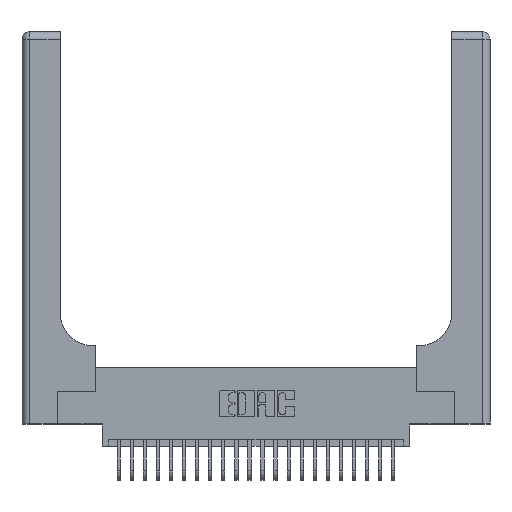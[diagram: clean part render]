
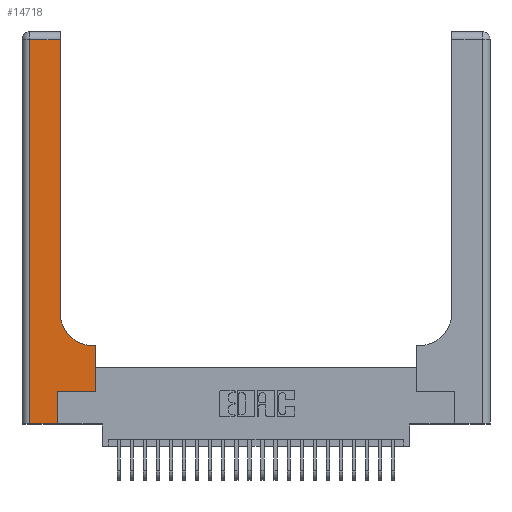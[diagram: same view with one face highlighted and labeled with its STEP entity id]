
A CAD part, top view. The second image highlights one B-rep face of the part: STEP entity #14718.
In plain terms, the highlighted planar face has unit normal (0, 0, 1).
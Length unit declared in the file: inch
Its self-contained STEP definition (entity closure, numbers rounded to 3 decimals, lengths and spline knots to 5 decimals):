
#81 = EDGE_CURVE ( 'NONE', #1444, #2046, #4703, .T. ) ;
#91 = VERTEX_POINT ( 'NONE', #6075 ) ;
#404 = VERTEX_POINT ( 'NONE', #10961 ) ;
#460 = AXIS2_PLACEMENT_3D ( 'NONE', #19530, #2668, #13280 ) ;
#1037 = ORIENTED_EDGE ( 'NONE', *, *, #14187, .T. ) ;
#1044 = FACE_OUTER_BOUND ( 'NONE', #12838, .T. ) ;
#1063 = ORIENTED_EDGE ( 'NONE', *, *, #23342, .T. ) ;
#1372 = CARTESIAN_POINT ( 'NONE',  ( 0., 0., 0.37 ) ) ;
#1444 = VERTEX_POINT ( 'NONE', #19657 ) ;
#1513 = DIRECTION ( 'NONE',  ( 1., 0., 0. ) ) ;
#2046 = VERTEX_POINT ( 'NONE', #17172 ) ;
#2134 = VECTOR ( 'NONE', #10286, 39.37008 ) ;
#2164 = ORIENTED_EDGE ( 'NONE', *, *, #81, .T. ) ;
#2668 = DIRECTION ( 'NONE',  ( 0., 0., -1. ) ) ;
#2847 = CARTESIAN_POINT ( 'NONE',  ( 0.269, 0.25, 0.37 ) ) ;
#3532 = VECTOR ( 'NONE', #17425, 39.37008 ) ;
#4218 = LINE ( 'NONE', #2847, #19525 ) ;
#4459 = ORIENTED_EDGE ( 'NONE', *, *, #10634, .T. ) ;
#4656 = LINE ( 'NONE', #13996, #14428 ) ;
#4703 = LINE ( 'NONE', #25936, #19701 ) ;
#5780 = EDGE_CURVE ( 'NONE', #404, #91, #26112, .T. ) ;
#6016 = CARTESIAN_POINT ( 'NONE',  ( 0.2915, 0.85, 0.37 ) ) ;
#6075 = CARTESIAN_POINT ( 'NONE',  ( 0.06, 2.94, 0.37 ) ) ;
#6311 = PLANE ( 'NONE',  #460 ) ;
#7303 = CARTESIAN_POINT ( 'NONE',  ( 0.2915, 3., 0.37 ) ) ;
#7791 = DIRECTION ( 'NONE',  ( 0., 1., 0. ) ) ;
#9221 = ORIENTED_EDGE ( 'NONE', *, *, #11347, .T. ) ;
#9480 = CARTESIAN_POINT ( 'NONE',  ( 0., 2.94, 0.37 ) ) ;
#9485 = AXIS2_PLACEMENT_3D ( 'NONE', #26447, #13960, #1513 ) ;
#10286 = DIRECTION ( 'NONE',  ( 0., 1., 0. ) ) ;
#10455 = CARTESIAN_POINT ( 'NONE',  ( 0.269, 0., 0.37 ) ) ;
#10634 = EDGE_CURVE ( 'NONE', #19384, #22992, #16503, .T. ) ;
#10961 = CARTESIAN_POINT ( 'NONE',  ( 0.2915, 2.94, 0.37 ) ) ;
#11347 = EDGE_CURVE ( 'NONE', #19010, #404, #17881, .T. ) ;
#11810 = VERTEX_POINT ( 'NONE', #13758 ) ;
#12633 = CARTESIAN_POINT ( 'NONE',  ( 0.06, 3., 0.37 ) ) ;
#12838 = EDGE_LOOP ( 'NONE', ( #9221, #25939, #1063, #18728, #4459, #26651, #1037, #2164, #24105 ) ) ;
#12932 = VECTOR ( 'NONE', #13661, 39.37008 ) ;
#13149 = DIRECTION ( 'NONE',  ( -1., 0., 0. ) ) ;
#13280 = DIRECTION ( 'NONE',  ( -1., 0., 0. ) ) ;
#13661 = DIRECTION ( 'NONE',  ( 0., 1., 0. ) ) ;
#13758 = CARTESIAN_POINT ( 'NONE',  ( 0.06, 0., 0.37 ) ) ;
#13960 = DIRECTION ( 'NONE',  ( 0., 0., -1. ) ) ;
#13996 = CARTESIAN_POINT ( 'NONE',  ( 0.5585, 0.25, 0.37 ) ) ;
#14081 = CIRCLE ( 'NONE', #9485, 0.25 ) ;
#14187 = EDGE_CURVE ( 'NONE', #15888, #1444, #4656, .T. ) ;
#14428 = VECTOR ( 'NONE', #7791, 39.37008 ) ;
#14685 = EDGE_CURVE ( 'NONE', #2046, #19010, #14081, .T. ) ;
#14718 = ADVANCED_FACE ( 'NONE', ( #1044 ), #6311, .F. ) ;
#15100 = DIRECTION ( 'NONE',  ( 1., 0., 0. ) ) ;
#15777 = LINE ( 'NONE', #1372, #20692 ) ;
#15888 = VERTEX_POINT ( 'NONE', #23251 ) ;
#16503 = LINE ( 'NONE', #10455, #2134 ) ;
#17172 = CARTESIAN_POINT ( 'NONE',  ( 0.5415, 0.6, 0.37 ) ) ;
#17425 = DIRECTION ( 'NONE',  ( 0., -1., 0. ) ) ;
#17881 = LINE ( 'NONE', #7303, #12932 ) ;
#18158 = DIRECTION ( 'NONE',  ( 1., 0., 0. ) ) ;
#18728 = ORIENTED_EDGE ( 'NONE', *, *, #25443, .T. ) ;
#19010 = VERTEX_POINT ( 'NONE', #6016 ) ;
#19384 = VERTEX_POINT ( 'NONE', #22228 ) ;
#19525 = VECTOR ( 'NONE', #15100, 39.37008 ) ;
#19530 = CARTESIAN_POINT ( 'NONE',  ( 0., 3., 0.37 ) ) ;
#19657 = CARTESIAN_POINT ( 'NONE',  ( 0.5585, 0.6, 0.37 ) ) ;
#19701 = VECTOR ( 'NONE', #13149, 39.37008 ) ;
#19937 = VECTOR ( 'NONE', #26178, 39.37008 ) ;
#20692 = VECTOR ( 'NONE', #18158, 39.37008 ) ;
#22228 = CARTESIAN_POINT ( 'NONE',  ( 0.269, 0., 0.37 ) ) ;
#22407 = EDGE_CURVE ( 'NONE', #22992, #15888, #4218, .T. ) ;
#22992 = VERTEX_POINT ( 'NONE', #23401 ) ;
#23251 = CARTESIAN_POINT ( 'NONE',  ( 0.5585, 0.25, 0.37 ) ) ;
#23342 = EDGE_CURVE ( 'NONE', #91, #11810, #25316, .T. ) ;
#23401 = CARTESIAN_POINT ( 'NONE',  ( 0.269, 0.25, 0.37 ) ) ;
#24105 = ORIENTED_EDGE ( 'NONE', *, *, #14685, .T. ) ;
#25316 = LINE ( 'NONE', #12633, #3532 ) ;
#25443 = EDGE_CURVE ( 'NONE', #11810, #19384, #15777, .T. ) ;
#25936 = CARTESIAN_POINT ( 'NONE',  ( 0.2915, 0.6, 0.37 ) ) ;
#25939 = ORIENTED_EDGE ( 'NONE', *, *, #5780, .T. ) ;
#26112 = LINE ( 'NONE', #9480, #19937 ) ;
#26178 = DIRECTION ( 'NONE',  ( -1., 0., 0. ) ) ;
#26447 = CARTESIAN_POINT ( 'NONE',  ( 0.5415, 0.85, 0.37 ) ) ;
#26651 = ORIENTED_EDGE ( 'NONE', *, *, #22407, .T. ) ;
